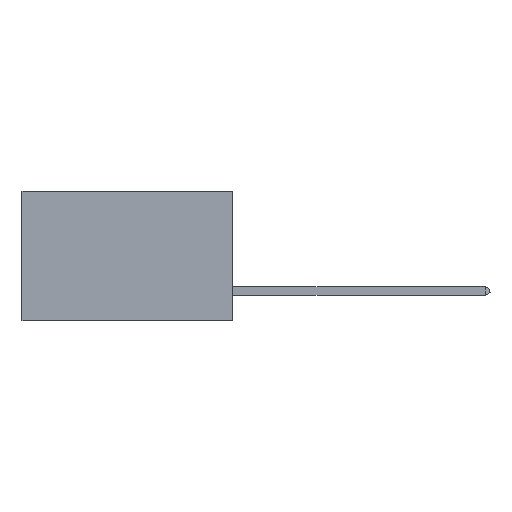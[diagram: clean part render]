
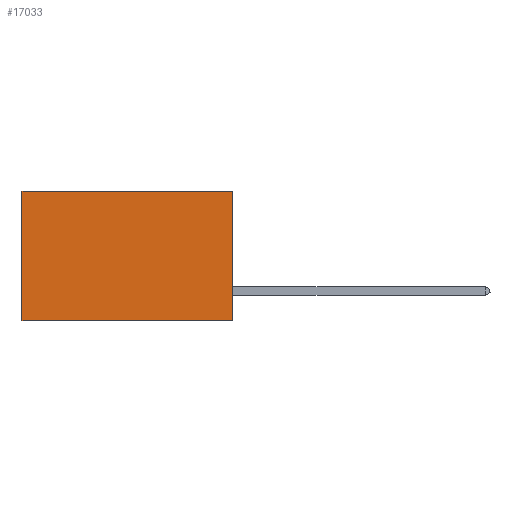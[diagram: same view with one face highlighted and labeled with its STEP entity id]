
A CAD part, left-side view. The second image highlights one B-rep face of the part: STEP entity #17033.
In plain terms, the highlighted planar face has unit normal (-1, 0, 0).
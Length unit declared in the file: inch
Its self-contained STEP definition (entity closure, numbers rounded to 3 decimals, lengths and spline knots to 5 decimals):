
#80 = FACE_OUTER_BOUND ( 'NONE', #21741, .T. ) ;
#475 = CARTESIAN_POINT ( 'NONE',  ( 0.2875, 0., 0. ) ) ;
#747 = VECTOR ( 'NONE', #19615, 39.37008 ) ;
#761 = LINE ( 'NONE', #13694, #6842 ) ;
#1000 = LINE ( 'NONE', #21200, #747 ) ;
#1943 = ORIENTED_EDGE ( 'NONE', *, *, #1954, .T. ) ;
#1954 = EDGE_CURVE ( 'NONE', #20942, #7213, #1000, .T. ) ;
#4426 = LINE ( 'NONE', #22222, #13239 ) ;
#5120 = DIRECTION ( 'NONE',  ( 0., 0., -1. ) ) ;
#5210 = CARTESIAN_POINT ( 'NONE',  ( 0.2875, 0., 0. ) ) ;
#5415 = CARTESIAN_POINT ( 'NONE',  ( 0.2875, 0.6, -0.37 ) ) ;
#6842 = VECTOR ( 'NONE', #5120, 39.37008 ) ;
#6940 = CARTESIAN_POINT ( 'NONE',  ( 0.2875, 0.6, 0. ) ) ;
#7213 = VERTEX_POINT ( 'NONE', #5415 ) ;
#7261 = LINE ( 'NONE', #5210, #18738 ) ;
#7386 = CARTESIAN_POINT ( 'NONE',  ( 0.2875, 0., 0. ) ) ;
#7805 = EDGE_CURVE ( 'NONE', #10215, #7213, #4426, .T. ) ;
#9823 = DIRECTION ( 'NONE',  ( 0., 1., 0. ) ) ;
#10003 = EDGE_CURVE ( 'NONE', #14384, #20942, #7261, .T. ) ;
#10211 = CARTESIAN_POINT ( 'NONE',  ( 0.2875, 0., -0.37 ) ) ;
#10215 = VERTEX_POINT ( 'NONE', #10211 ) ;
#10734 = ORIENTED_EDGE ( 'NONE', *, *, #13709, .F. ) ;
#13239 = VECTOR ( 'NONE', #9823, 39.37008 ) ;
#13694 = CARTESIAN_POINT ( 'NONE',  ( 0.2875, 0., 0. ) ) ;
#13709 = EDGE_CURVE ( 'NONE', #14384, #10215, #761, .T. ) ;
#14226 = AXIS2_PLACEMENT_3D ( 'NONE', #7386, #16291, #14628 ) ;
#14384 = VERTEX_POINT ( 'NONE', #475 ) ;
#14628 = DIRECTION ( 'NONE',  ( 0., 0., -1. ) ) ;
#16141 = ORIENTED_EDGE ( 'NONE', *, *, #10003, .T. ) ;
#16291 = DIRECTION ( 'NONE',  ( 1., 0., 0. ) ) ;
#17033 = ADVANCED_FACE ( 'NONE', ( #80 ), #19760, .F. ) ;
#17599 = ORIENTED_EDGE ( 'NONE', *, *, #7805, .F. ) ;
#18085 = DIRECTION ( 'NONE',  ( 0., 1., 0. ) ) ;
#18738 = VECTOR ( 'NONE', #18085, 39.37008 ) ;
#19615 = DIRECTION ( 'NONE',  ( 0., 0., -1. ) ) ;
#19760 = PLANE ( 'NONE',  #14226 ) ;
#20942 = VERTEX_POINT ( 'NONE', #6940 ) ;
#21200 = CARTESIAN_POINT ( 'NONE',  ( 0.2875, 0.6, 0. ) ) ;
#21741 = EDGE_LOOP ( 'NONE', ( #1943, #17599, #10734, #16141 ) ) ;
#22222 = CARTESIAN_POINT ( 'NONE',  ( 0.2875, 0., -0.37 ) ) ;
